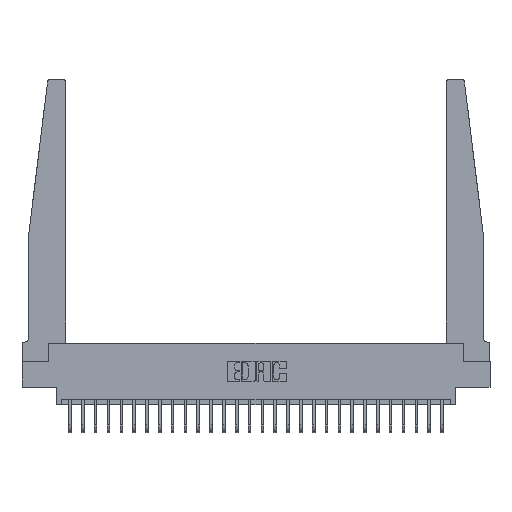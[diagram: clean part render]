
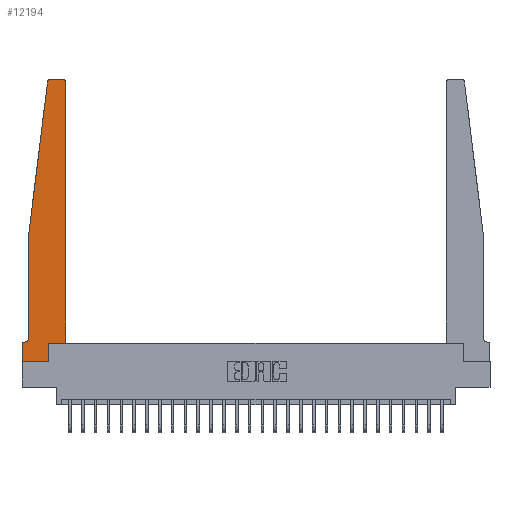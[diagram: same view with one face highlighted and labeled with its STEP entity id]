
A CAD part, top view. The second image highlights one B-rep face of the part: STEP entity #12194.
In plain terms, the highlighted planar face has unit normal (0, 0, 1).
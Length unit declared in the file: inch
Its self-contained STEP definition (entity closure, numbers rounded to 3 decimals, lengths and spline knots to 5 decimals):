
#38 = ORIENTED_EDGE ( 'NONE', *, *, #595, .T. ) ;
#595 = EDGE_CURVE ( 'NONE', #23702, #6959, #11824, .T. ) ;
#843 = CARTESIAN_POINT ( 'NONE',  ( 0.25, 2.75, 0.37 ) ) ;
#1190 = VERTEX_POINT ( 'NONE', #10898 ) ;
#1674 = CARTESIAN_POINT ( 'NONE',  ( 0.065, 1.25, 0.37 ) ) ;
#1715 = LINE ( 'NONE', #3655, #2337 ) ;
#2044 = VECTOR ( 'NONE', #3415, 39.37008 ) ;
#2198 = CIRCLE ( 'NONE', #16413, 0.05 ) ;
#2203 = CARTESIAN_POINT ( 'NONE',  ( 0.065, 1.25, 0.37 ) ) ;
#2226 = CARTESIAN_POINT ( 'NONE',  ( 0., 0., 0.37 ) ) ;
#2337 = VECTOR ( 'NONE', #15295, 39.37008 ) ;
#2485 = DIRECTION ( 'NONE',  ( 0., 0., -1. ) ) ;
#2670 = EDGE_CURVE ( 'NONE', #3138, #1190, #15803, .T. ) ;
#3138 = VERTEX_POINT ( 'NONE', #22043 ) ;
#3415 = DIRECTION ( 'NONE',  ( 0., 1., 0. ) ) ;
#3655 = CARTESIAN_POINT ( 'NONE',  ( 0.425, 0.18, 0.37 ) ) ;
#3678 = DIRECTION ( 'NONE',  ( 1., 0., 0. ) ) ;
#5123 = CARTESIAN_POINT ( 'NONE',  ( 0.27653, 2.72, 0.37 ) ) ;
#5456 = VECTOR ( 'NONE', #18638, 39.37008 ) ;
#5976 = VERTEX_POINT ( 'NONE', #25059 ) ;
#6006 = VERTEX_POINT ( 'NONE', #7752 ) ;
#6498 = AXIS2_PLACEMENT_3D ( 'NONE', #13366, #15319, #3678 ) ;
#6959 = VERTEX_POINT ( 'NONE', #22393 ) ;
#7081 = DIRECTION ( 'NONE',  ( 1., 0., 0. ) ) ;
#7314 = EDGE_CURVE ( 'NONE', #23766, #3138, #2198, .T. ) ;
#7507 = EDGE_CURVE ( 'NONE', #23804, #24405, #8314, .T. ) ;
#7510 = PLANE ( 'NONE',  #6498 ) ;
#7739 = CARTESIAN_POINT ( 'NONE',  ( 0., 0., 0.37 ) ) ;
#7752 = CARTESIAN_POINT ( 'NONE',  ( 0.395, 2.75, 0.37 ) ) ;
#7910 = CARTESIAN_POINT ( 'NONE',  ( 0., 0., 0.37 ) ) ;
#8044 = LINE ( 'NONE', #7739, #14417 ) ;
#8206 = LINE ( 'NONE', #20300, #23093 ) ;
#8314 = LINE ( 'NONE', #7910, #8923 ) ;
#8633 = DIRECTION ( 'NONE',  ( -1., 0., 0. ) ) ;
#8835 = CARTESIAN_POINT ( 'NONE',  ( 0.065, 0.1875, 0.37 ) ) ;
#8839 = VERTEX_POINT ( 'NONE', #12180 ) ;
#8923 = VECTOR ( 'NONE', #13762, 39.37008 ) ;
#9293 = CIRCLE ( 'NONE', #21168, 0.03 ) ;
#9546 = ORIENTED_EDGE ( 'NONE', *, *, #12047, .T. ) ;
#9562 = DIRECTION ( 'NONE',  ( 0., 0., 1. ) ) ;
#10419 = EDGE_CURVE ( 'NONE', #6959, #6006, #9293, .T. ) ;
#10898 = CARTESIAN_POINT ( 'NONE',  ( 0., 0.1875, 0.37 ) ) ;
#10965 = EDGE_CURVE ( 'NONE', #1190, #23804, #8044, .T. ) ;
#11163 = ORIENTED_EDGE ( 'NONE', *, *, #17912, .T. ) ;
#11398 = ORIENTED_EDGE ( 'NONE', *, *, #19528, .T. ) ;
#11679 = EDGE_LOOP ( 'NONE', ( #24350, #9546, #11398, #11163, #17112, #13241, #19855, #22998, #18590, #13876, #38, #17940 ) ) ;
#11824 = LINE ( 'NONE', #15045, #2044 ) ;
#11917 = EDGE_CURVE ( 'NONE', #6006, #19831, #17135, .T. ) ;
#12047 = EDGE_CURVE ( 'NONE', #19831, #19542, #24986, .T. ) ;
#12180 = CARTESIAN_POINT ( 'NONE',  ( 0.065, 1.25, 0.37 ) ) ;
#12194 = ADVANCED_FACE ( 'NONE', ( #20755 ), #7510, .T. ) ;
#12850 = CARTESIAN_POINT ( 'NONE',  ( 0.27653, 2.75, 0.37 ) ) ;
#13241 = ORIENTED_EDGE ( 'NONE', *, *, #2670, .T. ) ;
#13366 = CARTESIAN_POINT ( 'NONE',  ( 0., 0.1875, 0.37 ) ) ;
#13531 = AXIS2_PLACEMENT_3D ( 'NONE', #5123, #18766, #7081 ) ;
#13762 = DIRECTION ( 'NONE',  ( 1., 0., 0. ) ) ;
#13876 = ORIENTED_EDGE ( 'NONE', *, *, #22977, .T. ) ;
#14131 = CARTESIAN_POINT ( 'NONE',  ( 0.015, 0.2375, 0.37 ) ) ;
#14396 = DIRECTION ( 'NONE',  ( 0., 1., 0. ) ) ;
#14417 = VECTOR ( 'NONE', #21338, 39.37008 ) ;
#15045 = CARTESIAN_POINT ( 'NONE',  ( 0.425, 0.18, 0.37 ) ) ;
#15295 = DIRECTION ( 'NONE',  ( 1., 0., 0. ) ) ;
#15319 = DIRECTION ( 'NONE',  ( 0., 0., 1. ) ) ;
#15425 = CARTESIAN_POINT ( 'NONE',  ( 0.425, 0.18, 0.37 ) ) ;
#15803 = LINE ( 'NONE', #8835, #5456 ) ;
#16106 = DIRECTION ( 'NONE',  ( -1., 0., 0. ) ) ;
#16413 = AXIS2_PLACEMENT_3D ( 'NONE', #14131, #2485, #16106 ) ;
#17112 = ORIENTED_EDGE ( 'NONE', *, *, #7314, .T. ) ;
#17135 = LINE ( 'NONE', #843, #21658 ) ;
#17674 = CARTESIAN_POINT ( 'NONE',  ( 0.065, 0.2375, 0.37 ) ) ;
#17713 = LINE ( 'NONE', #2203, #22222 ) ;
#17817 = DIRECTION ( 'NONE',  ( -0.122, -0.992, 0. ) ) ;
#17898 = CARTESIAN_POINT ( 'NONE',  ( 0.24675, 2.72367, 0.37 ) ) ;
#17912 = EDGE_CURVE ( 'NONE', #8839, #23766, #22612, .T. ) ;
#17940 = ORIENTED_EDGE ( 'NONE', *, *, #10419, .T. ) ;
#18590 = ORIENTED_EDGE ( 'NONE', *, *, #22041, .T. ) ;
#18638 = DIRECTION ( 'NONE',  ( -1., 0., 0. ) ) ;
#18718 = VECTOR ( 'NONE', #21025, 39.37008 ) ;
#18766 = DIRECTION ( 'NONE',  ( 0., 0., 1. ) ) ;
#19528 = EDGE_CURVE ( 'NONE', #19542, #8839, #17713, .T. ) ;
#19542 = VERTEX_POINT ( 'NONE', #17898 ) ;
#19831 = VERTEX_POINT ( 'NONE', #12850 ) ;
#19855 = ORIENTED_EDGE ( 'NONE', *, *, #10965, .T. ) ;
#20273 = CARTESIAN_POINT ( 'NONE',  ( 0.2605, 0., 0.37 ) ) ;
#20300 = CARTESIAN_POINT ( 'NONE',  ( 0.2605, 0.18, 0.37 ) ) ;
#20755 = FACE_OUTER_BOUND ( 'NONE', #11679, .T. ) ;
#21025 = DIRECTION ( 'NONE',  ( 0., -1., 0. ) ) ;
#21168 = AXIS2_PLACEMENT_3D ( 'NONE', #21188, #9562, #23134 ) ;
#21188 = CARTESIAN_POINT ( 'NONE',  ( 0.395, 2.72, 0.37 ) ) ;
#21338 = DIRECTION ( 'NONE',  ( 0., -1., 0. ) ) ;
#21658 = VECTOR ( 'NONE', #8633, 39.37008 ) ;
#22041 = EDGE_CURVE ( 'NONE', #24405, #5976, #8206, .T. ) ;
#22043 = CARTESIAN_POINT ( 'NONE',  ( 0.015, 0.1875, 0.37 ) ) ;
#22222 = VECTOR ( 'NONE', #17817, 39.37008 ) ;
#22393 = CARTESIAN_POINT ( 'NONE',  ( 0.425, 2.72, 0.37 ) ) ;
#22612 = LINE ( 'NONE', #1674, #18718 ) ;
#22977 = EDGE_CURVE ( 'NONE', #5976, #23702, #1715, .T. ) ;
#22998 = ORIENTED_EDGE ( 'NONE', *, *, #7507, .T. ) ;
#23093 = VECTOR ( 'NONE', #14396, 39.37008 ) ;
#23134 = DIRECTION ( 'NONE',  ( 1., 0., 0. ) ) ;
#23702 = VERTEX_POINT ( 'NONE', #15425 ) ;
#23766 = VERTEX_POINT ( 'NONE', #17674 ) ;
#23804 = VERTEX_POINT ( 'NONE', #2226 ) ;
#24350 = ORIENTED_EDGE ( 'NONE', *, *, #11917, .T. ) ;
#24405 = VERTEX_POINT ( 'NONE', #20273 ) ;
#24986 = CIRCLE ( 'NONE', #13531, 0.03 ) ;
#25059 = CARTESIAN_POINT ( 'NONE',  ( 0.2605, 0.18, 0.37 ) ) ;
